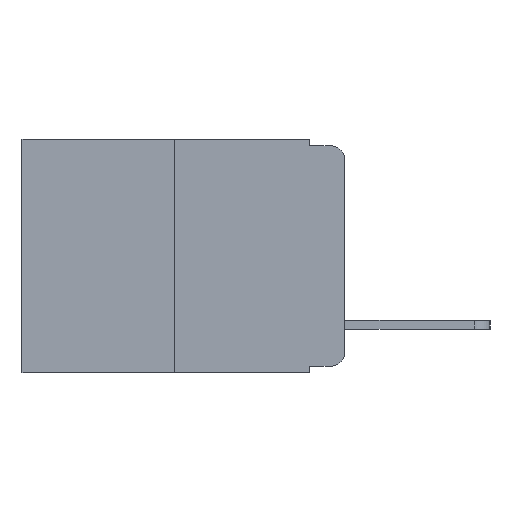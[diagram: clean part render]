
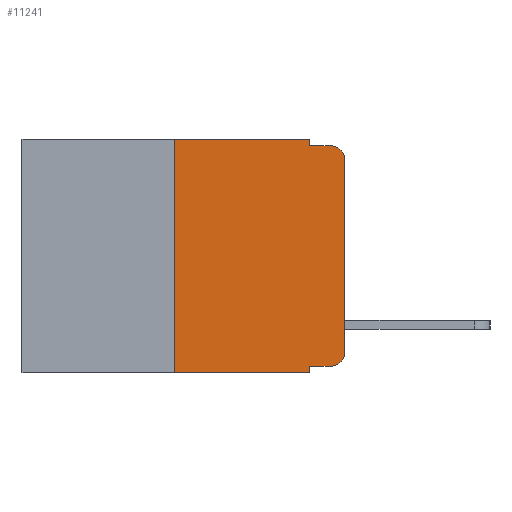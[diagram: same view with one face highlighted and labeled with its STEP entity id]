
A CAD part, left-side view. The second image highlights one B-rep face of the part: STEP entity #11241.
In plain terms, the highlighted planar face has unit normal (-1, 0, 0).
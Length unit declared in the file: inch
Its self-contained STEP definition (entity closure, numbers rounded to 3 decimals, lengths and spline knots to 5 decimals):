
#30 = VERTEX_POINT ( 'NONE', #4481 ) ;
#132 = CARTESIAN_POINT ( 'NONE',  ( 0., 0.051, 0. ) ) ;
#1040 = VERTEX_POINT ( 'NONE', #8568 ) ;
#1131 = LINE ( 'NONE', #12075, #15292 ) ;
#1623 = VERTEX_POINT ( 'NONE', #14640 ) ;
#1727 = DIRECTION ( 'NONE',  ( 0., 0., -1. ) ) ;
#1753 = CARTESIAN_POINT ( 'NONE',  ( 0., 0.25, -0.343 ) ) ;
#1861 = DIRECTION ( 'NONE',  ( 0., -1., 0. ) ) ;
#1902 = CARTESIAN_POINT ( 'NONE',  ( 0., 0.051, -0.343 ) ) ;
#2301 = DIRECTION ( 'NONE',  ( 0., 0., 1. ) ) ;
#2444 = DIRECTION ( 'NONE',  ( 0., 0., -1. ) ) ;
#2450 = CIRCLE ( 'NONE', #17417, 0.02 ) ;
#2522 = VECTOR ( 'NONE', #11917, 39.37008 ) ;
#2614 = CARTESIAN_POINT ( 'NONE',  ( 0., 0.473, 0. ) ) ;
#2630 = VERTEX_POINT ( 'NONE', #8339 ) ;
#2761 = CARTESIAN_POINT ( 'NONE',  ( 0., 0., -0.03 ) ) ;
#2784 = LINE ( 'NONE', #2614, #10320 ) ;
#2915 = DIRECTION ( 'NONE',  ( 0., 0., 1. ) ) ;
#3570 = CARTESIAN_POINT ( 'NONE',  ( 0., 0.051, 0. ) ) ;
#3714 = VERTEX_POINT ( 'NONE', #10499 ) ;
#3719 = AXIS2_PLACEMENT_3D ( 'NONE', #12225, #3979, #13476 ) ;
#3823 = LINE ( 'NONE', #16577, #7546 ) ;
#3869 = VERTEX_POINT ( 'NONE', #1902 ) ;
#3979 = DIRECTION ( 'NONE',  ( -1., 0., 0. ) ) ;
#4481 = CARTESIAN_POINT ( 'NONE',  ( 0., 0.051, 0. ) ) ;
#4584 = VERTEX_POINT ( 'NONE', #2761 ) ;
#5144 = EDGE_CURVE ( 'NONE', #12083, #30, #2784, .T. ) ;
#5244 = DIRECTION ( 'NONE',  ( 0., -1., 0. ) ) ;
#5456 = VECTOR ( 'NONE', #2915, 39.37008 ) ;
#5536 = ORIENTED_EDGE ( 'NONE', *, *, #15621, .T. ) ;
#5810 = ORIENTED_EDGE ( 'NONE', *, *, #14805, .T. ) ;
#6004 = ORIENTED_EDGE ( 'NONE', *, *, #14001, .F. ) ;
#6102 = ORIENTED_EDGE ( 'NONE', *, *, #12340, .F. ) ;
#6300 = LINE ( 'NONE', #132, #13045 ) ;
#6371 = VECTOR ( 'NONE', #6460, 39.37008 ) ;
#6460 = DIRECTION ( 'NONE',  ( 0., 0., -1. ) ) ;
#6696 = ORIENTED_EDGE ( 'NONE', *, *, #5144, .F. ) ;
#6790 = ORIENTED_EDGE ( 'NONE', *, *, #11479, .F. ) ;
#6942 = ORIENTED_EDGE ( 'NONE', *, *, #12569, .T. ) ;
#7031 = ORIENTED_EDGE ( 'NONE', *, *, #10566, .F. ) ;
#7071 = ORIENTED_EDGE ( 'NONE', *, *, #9661, .T. ) ;
#7131 = AXIS2_PLACEMENT_3D ( 'NONE', #13469, #10958, #2444 ) ;
#7200 = ORIENTED_EDGE ( 'NONE', *, *, #7770, .T. ) ;
#7546 = VECTOR ( 'NONE', #11639, 39.37008 ) ;
#7554 = VECTOR ( 'NONE', #2301, 39.37008 ) ;
#7770 = EDGE_CURVE ( 'NONE', #7798, #3714, #2450, .T. ) ;
#7798 = VERTEX_POINT ( 'NONE', #11393 ) ;
#8339 = CARTESIAN_POINT ( 'NONE',  ( 0., 0.051, -0.01 ) ) ;
#8568 = CARTESIAN_POINT ( 'NONE',  ( 0., 0.051, -0.333 ) ) ;
#9661 = EDGE_CURVE ( 'NONE', #1040, #7798, #3823, .T. ) ;
#9992 = CARTESIAN_POINT ( 'NONE',  ( 0., 0.25, 0. ) ) ;
#10020 = LINE ( 'NONE', #3570, #6371 ) ;
#10320 = VECTOR ( 'NONE', #1861, 39.37008 ) ;
#10499 = CARTESIAN_POINT ( 'NONE',  ( 0., 0., -0.313 ) ) ;
#10561 = CARTESIAN_POINT ( 'NONE',  ( 0., 0.051, -0.01 ) ) ;
#10566 = EDGE_CURVE ( 'NONE', #1040, #3869, #10020, .T. ) ;
#10817 = CARTESIAN_POINT ( 'NONE',  ( 0., 0., 0. ) ) ;
#10958 = DIRECTION ( 'NONE',  ( 1., 0., 0. ) ) ;
#11241 = ADVANCED_FACE ( 'NONE', ( #15339 ), #15888, .F. ) ;
#11354 = CIRCLE ( 'NONE', #3719, 0.02 ) ;
#11393 = CARTESIAN_POINT ( 'NONE',  ( 0., 0.02, -0.333 ) ) ;
#11479 = EDGE_CURVE ( 'NONE', #11716, #12083, #15530, .T. ) ;
#11639 = DIRECTION ( 'NONE',  ( 0., -1., 0. ) ) ;
#11716 = VERTEX_POINT ( 'NONE', #1753 ) ;
#11917 = DIRECTION ( 'NONE',  ( 0., -1., 0. ) ) ;
#11956 = LINE ( 'NONE', #10817, #7554 ) ;
#12075 = CARTESIAN_POINT ( 'NONE',  ( 0., 0.473, -0.343 ) ) ;
#12083 = VERTEX_POINT ( 'NONE', #17312 ) ;
#12225 = CARTESIAN_POINT ( 'NONE',  ( 0., 0.02, -0.03 ) ) ;
#12340 = EDGE_CURVE ( 'NONE', #30, #2630, #6300, .T. ) ;
#12569 = EDGE_CURVE ( 'NONE', #11716, #3869, #1131, .T. ) ;
#12822 = DIRECTION ( 'NONE',  ( 0., 0., -1. ) ) ;
#13000 = DIRECTION ( 'NONE',  ( -1., 0., 0. ) ) ;
#13043 = CARTESIAN_POINT ( 'NONE',  ( 0., 0.02, -0.313 ) ) ;
#13045 = VECTOR ( 'NONE', #1727, 39.37008 ) ;
#13187 = LINE ( 'NONE', #10561, #2522 ) ;
#13215 = EDGE_LOOP ( 'NONE', ( #5536, #5810, #6004, #6102, #6696, #6790, #6942, #7031, #7071, #7200 ) ) ;
#13469 = CARTESIAN_POINT ( 'NONE',  ( 0., 0.473, 0. ) ) ;
#13476 = DIRECTION ( 'NONE',  ( 0., 0., -1. ) ) ;
#14001 = EDGE_CURVE ( 'NONE', #2630, #1623, #13187, .T. ) ;
#14640 = CARTESIAN_POINT ( 'NONE',  ( 0., 0.02, -0.01 ) ) ;
#14805 = EDGE_CURVE ( 'NONE', #4584, #1623, #11354, .T. ) ;
#15292 = VECTOR ( 'NONE', #5244, 39.37008 ) ;
#15339 = FACE_OUTER_BOUND ( 'NONE', #13215, .T. ) ;
#15530 = LINE ( 'NONE', #9992, #5456 ) ;
#15621 = EDGE_CURVE ( 'NONE', #3714, #4584, #11956, .T. ) ;
#15888 = PLANE ( 'NONE',  #7131 ) ;
#16577 = CARTESIAN_POINT ( 'NONE',  ( 0., 0.051, -0.333 ) ) ;
#17312 = CARTESIAN_POINT ( 'NONE',  ( 0., 0.25, 0. ) ) ;
#17417 = AXIS2_PLACEMENT_3D ( 'NONE', #13043, #13000, #12822 ) ;
